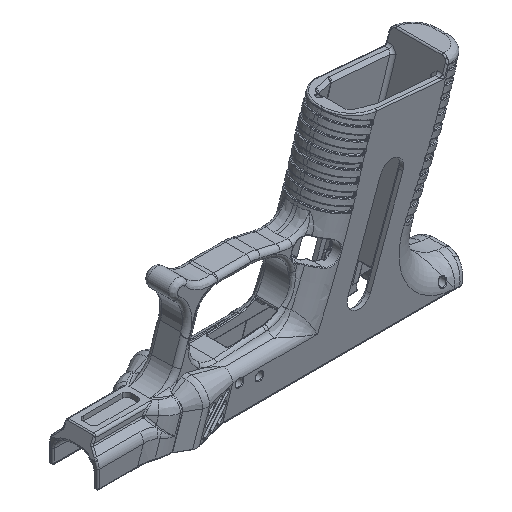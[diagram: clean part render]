
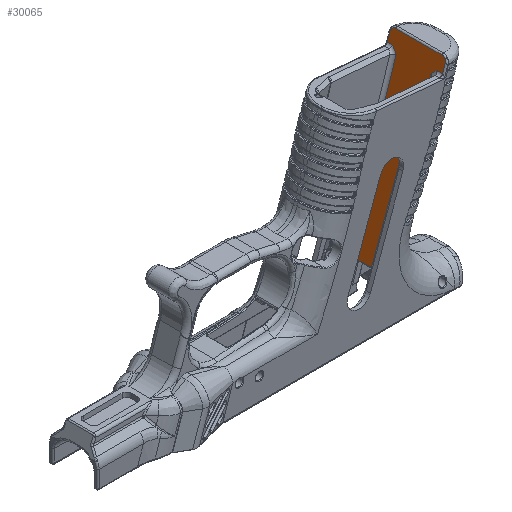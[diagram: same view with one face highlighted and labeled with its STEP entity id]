
A CAD part, isometric view. The second image highlights one B-rep face of the part: STEP entity #30065.
In plain terms, the highlighted planar face has unit normal (-0.951, 0, 0.309).
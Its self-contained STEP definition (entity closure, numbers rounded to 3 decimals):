
#643=B_SPLINE_CURVE_WITH_KNOTS('',3,(#64669,#64670,#64671,#64672),
 .UNSPECIFIED.,.F.,.F.,(4,4),(0.135,0.185),
 .UNSPECIFIED.);
#648=B_SPLINE_CURVE_WITH_KNOTS('',3,(#64812,#64813,#64814,#64815),
 .UNSPECIFIED.,.F.,.F.,(4,4),(0.,0.151),.UNSPECIFIED.);
#1627=ELLIPSE('',#32515,1.618,1.385);
#1631=ELLIPSE('',#32523,0.503,0.422);
#1672=ELLIPSE('',#32916,1.903,1.854);
#1718=ELLIPSE('',#33189,1.903,1.854);
#6567=FACE_OUTER_BOUND('',#8583,.T.);
#8583=EDGE_LOOP('',(#25699,#25700,#25701,#25702,#25703,#25704,#25705,#25706,
#25707,#25708,#25709,#25710,#25711,#25712,#25713,#25714));
#10024=LINE('',#64643,#11358);
#10026=LINE('',#64680,#11360);
#10027=LINE('',#64686,#11361);
#10030=LINE('',#64726,#11364);
#10031=LINE('',#64730,#11365);
#10032=LINE('',#64736,#11366);
#10034=LINE('',#64767,#11368);
#10146=LINE('',#69068,#11480);
#10274=LINE('',#78701,#11608);
#10275=LINE('',#78703,#11609);
#11358=VECTOR('',#38776,0.33);
#11360=VECTOR('',#38784,10.);
#11361=VECTOR('',#38791,10.);
#11364=VECTOR('',#38806,10.);
#11365=VECTOR('',#38809,10.);
#11366=VECTOR('',#38818,10.);
#11368=VECTOR('',#38826,10.);
#11480=VECTOR('',#39394,10.);
#11608=VECTOR('',#40392,10.);
#11609=VECTOR('',#40395,10.);
#13036=VERTEX_POINT('',#54578);
#13223=VERTEX_POINT('',#57488);
#13499=VERTEX_POINT('',#64640);
#13500=VERTEX_POINT('',#64642);
#13503=VERTEX_POINT('',#64677);
#13504=VERTEX_POINT('',#64679);
#13506=VERTEX_POINT('',#64685);
#13509=VERTEX_POINT('',#64711);
#13511=VERTEX_POINT('',#64718);
#13512=VERTEX_POINT('',#64722);
#13514=VERTEX_POINT('',#64728);
#13515=VERTEX_POINT('',#64729);
#13518=VERTEX_POINT('',#64765);
#13522=VERTEX_POINT('',#64806);
#13823=VERTEX_POINT('',#73176);
#14031=VERTEX_POINT('',#78700);
#17130=EDGE_CURVE('',#13499,#13500,#10024,.T.);
#17132=EDGE_CURVE('',#13500,#13223,#643,.T.);
#17135=EDGE_CURVE('',#13503,#13504,#10026,.T.);
#17138=EDGE_CURVE('',#13504,#13506,#10027,.T.);
#17144=EDGE_CURVE('',#13511,#13509,#1627,.T.);
#17147=EDGE_CURVE('',#13509,#13512,#10030,.T.);
#17148=EDGE_CURVE('',#13514,#13515,#10031,.T.);
#17152=EDGE_CURVE('',#13515,#13036,#10032,.T.);
#17153=EDGE_CURVE('',#13036,#13499,#1631,.T.);
#17156=EDGE_CURVE('',#13518,#13514,#10034,.T.);
#17162=EDGE_CURVE('',#13512,#13522,#648,.T.);
#17479=EDGE_CURVE('',#13223,#13503,#10146,.T.);
#17736=EDGE_CURVE('',#13823,#13511,#1672,.T.);
#18119=EDGE_CURVE('',#14031,#13518,#10274,.T.);
#18120=EDGE_CURVE('',#13522,#14031,#1718,.T.);
#18121=EDGE_CURVE('',#13506,#13823,#10275,.T.);
#25699=ORIENTED_EDGE('',*,*,#17153,.F.);
#25700=ORIENTED_EDGE('',*,*,#17152,.F.);
#25701=ORIENTED_EDGE('',*,*,#17148,.F.);
#25702=ORIENTED_EDGE('',*,*,#17156,.F.);
#25703=ORIENTED_EDGE('',*,*,#18119,.F.);
#25704=ORIENTED_EDGE('',*,*,#18120,.F.);
#25705=ORIENTED_EDGE('',*,*,#17162,.F.);
#25706=ORIENTED_EDGE('',*,*,#17147,.F.);
#25707=ORIENTED_EDGE('',*,*,#17144,.F.);
#25708=ORIENTED_EDGE('',*,*,#17736,.F.);
#25709=ORIENTED_EDGE('',*,*,#18121,.F.);
#25710=ORIENTED_EDGE('',*,*,#17138,.F.);
#25711=ORIENTED_EDGE('',*,*,#17135,.F.);
#25712=ORIENTED_EDGE('',*,*,#17479,.F.);
#25713=ORIENTED_EDGE('',*,*,#17132,.F.);
#25714=ORIENTED_EDGE('',*,*,#17130,.F.);
#28555=PLANE('',#33188);
#30065=ADVANCED_FACE('',(#6567),#28555,.T.);
#32515=AXIS2_PLACEMENT_3D('',#64720,#38799,#38800);
#32523=AXIS2_PLACEMENT_3D('',#64761,#38819,#38820);
#32916=AXIS2_PLACEMENT_3D('',#73178,#39780,#39781);
#33188=AXIS2_PLACEMENT_3D('',#78699,#40390,#40391);
#33189=AXIS2_PLACEMENT_3D('',#78702,#40393,#40394);
#38776=DIRECTION('',(0.,1.,0.));
#38784=DIRECTION('',(0.221,0.698,0.681));
#38791=DIRECTION('',(0.,1.,0.));
#38799=DIRECTION('center_axis',(0.951,0.,
-0.309));
#38800=DIRECTION('ref_axis',(-0.138,0.895,-0.425));
#38806=DIRECTION('',(0.,-1.,0.));
#38809=DIRECTION('',(-0.221,0.698,-0.681));
#38818=DIRECTION('',(-0.309,0.,-0.951));
#38819=DIRECTION('center_axis',(-0.951,0.,
0.309));
#38820=DIRECTION('ref_axis',(-0.161,-0.853,-0.496));
#38826=DIRECTION('',(0.,1.,0.));
#39394=DIRECTION('',(0.309,0.,0.951));
#39780=DIRECTION('center_axis',(0.951,0.,-0.309));
#39781=DIRECTION('ref_axis',(0.309,0.,0.951));
#40390=DIRECTION('center_axis',(-0.951,0.,0.309));
#40391=DIRECTION('ref_axis',(0.309,0.,0.951));
#40392=DIRECTION('',(-0.309,0.,-0.951));
#40393=DIRECTION('center_axis',(0.951,0.,-0.309));
#40394=DIRECTION('ref_axis',(0.309,0.,0.951));
#40395=DIRECTION('',(0.309,0.,0.951));
#54578=CARTESIAN_POINT('',(45.003,-7.239,-14.987));
#57488=CARTESIAN_POINT('',(45.003,7.239,-14.987));
#64640=CARTESIAN_POINT('',(45.07,-6.795,-14.782));
#64642=CARTESIAN_POINT('',(45.07,6.795,-14.782));
#64643=CARTESIAN_POINT('',(45.07,0.,-14.782));
#64669=CARTESIAN_POINT('Ctrl Pts',(45.07,6.795,-14.782));
#64670=CARTESIAN_POINT('Ctrl Pts',(45.07,6.965,-14.782));
#64671=CARTESIAN_POINT('Ctrl Pts',(45.044,7.132,-14.862));
#64672=CARTESIAN_POINT('Ctrl Pts',(45.003,7.239,-14.987));
#64677=CARTESIAN_POINT('',(65.351,7.239,47.637));
#64679=CARTESIAN_POINT('',(65.989,9.253,49.603));
#64680=CARTESIAN_POINT('',(64.466,4.447,44.913));
#64685=CARTESIAN_POINT('',(65.989,11.557,49.603));
#64686=CARTESIAN_POINT('',(65.989,0.,49.603));
#64711=CARTESIAN_POINT('',(67.621,9.702,54.625));
#64718=CARTESIAN_POINT('',(67.438,11.047,54.062));
#64720=CARTESIAN_POINT('Origin',(67.178,9.897,53.261));
#64722=CARTESIAN_POINT('',(67.621,-9.702,54.625));
#64726=CARTESIAN_POINT('',(67.621,0.,54.625));
#64728=CARTESIAN_POINT('',(65.989,-9.253,49.603));
#64729=CARTESIAN_POINT('',(65.351,-7.239,47.637));
#64730=CARTESIAN_POINT('',(64.466,-4.447,44.913));
#64736=CARTESIAN_POINT('',(58.598,-7.239,26.855));
#64761=CARTESIAN_POINT('Origin',(44.932,-6.869,-15.205));
#64765=CARTESIAN_POINT('',(65.989,-11.557,49.603));
#64767=CARTESIAN_POINT('',(65.989,0.,49.603));
#64806=CARTESIAN_POINT('',(67.438,-11.047,54.062));
#64812=CARTESIAN_POINT('Ctrl Pts',(67.621,-9.702,54.625));
#64813=CARTESIAN_POINT('Ctrl Pts',(67.621,-10.206,54.625));
#64814=CARTESIAN_POINT('Ctrl Pts',(67.553,-10.704,54.414));
#64815=CARTESIAN_POINT('Ctrl Pts',(67.438,-11.047,54.062));
#69068=CARTESIAN_POINT('',(58.598,7.239,26.855));
#73176=CARTESIAN_POINT('',(67.033,11.557,52.816));
#73178=CARTESIAN_POINT('Origin',(67.033,9.703,52.816));
#78699=CARTESIAN_POINT('Origin',(65.677,0.,48.641));
#78700=CARTESIAN_POINT('',(67.033,-11.557,52.816));
#78701=CARTESIAN_POINT('',(57.252,-11.557,22.711));
#78702=CARTESIAN_POINT('Origin',(67.033,-9.703,52.816));
#78703=CARTESIAN_POINT('',(57.252,11.557,22.711));
